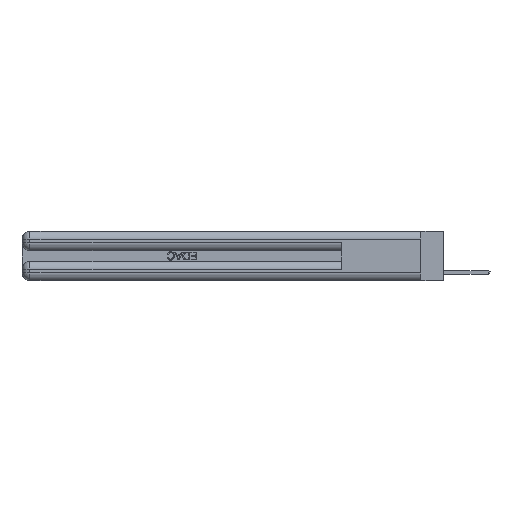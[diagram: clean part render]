
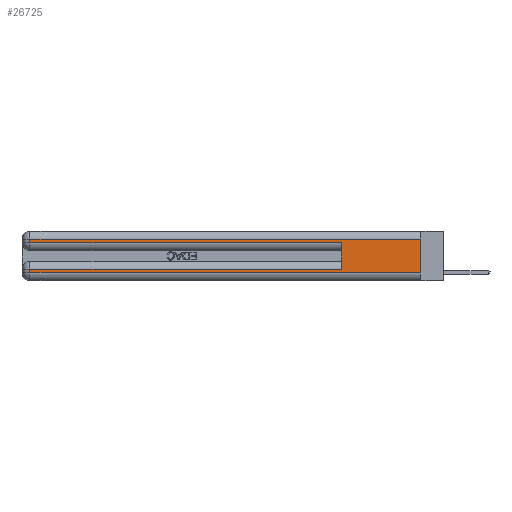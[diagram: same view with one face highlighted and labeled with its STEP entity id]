
A CAD part, left-side view. The second image highlights one B-rep face of the part: STEP entity #26725.
In plain terms, the highlighted planar face has unit normal (-1, 0, 0).
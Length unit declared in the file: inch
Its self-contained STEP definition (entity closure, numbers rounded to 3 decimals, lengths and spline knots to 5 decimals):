
#1378 = ORIENTED_EDGE ( 'NONE', *, *, #25001, .T. ) ;
#1379 = CARTESIAN_POINT ( 'NONE',  ( 0., 2.94, 0.06 ) ) ;
#1670 = ORIENTED_EDGE ( 'NONE', *, *, #17466, .T. ) ;
#1953 = VECTOR ( 'NONE', #6550, 39.37008 ) ;
#2352 = VERTEX_POINT ( 'NONE', #7837 ) ;
#2622 = DIRECTION ( 'NONE',  ( 0., 0., -1. ) ) ;
#2938 = PLANE ( 'NONE',  #23205 ) ;
#3796 = CARTESIAN_POINT ( 'NONE',  ( 0., 2.94, 0.31 ) ) ;
#4216 = VERTEX_POINT ( 'NONE', #20853 ) ;
#4381 = ORIENTED_EDGE ( 'NONE', *, *, #17596, .T. ) ;
#4648 = EDGE_CURVE ( 'NONE', #2352, #10303, #21858, .T. ) ;
#4790 = DIRECTION ( 'NONE',  ( 0., 0., -1. ) ) ;
#4871 = CARTESIAN_POINT ( 'NONE',  ( 0., 0., 0.37 ) ) ;
#5040 = ORIENTED_EDGE ( 'NONE', *, *, #4648, .T. ) ;
#5120 = LINE ( 'NONE', #5767, #29321 ) ;
#5767 = CARTESIAN_POINT ( 'NONE',  ( 0., 0., 0.06 ) ) ;
#6040 = VERTEX_POINT ( 'NONE', #1379 ) ;
#6550 = DIRECTION ( 'NONE',  ( 0., -1., 0. ) ) ;
#7837 = CARTESIAN_POINT ( 'NONE',  ( 0., 0., 0.31 ) ) ;
#8303 = VECTOR ( 'NONE', #22413, 39.37008 ) ;
#8618 = CARTESIAN_POINT ( 'NONE',  ( 0., 0., 0.085 ) ) ;
#8828 = CARTESIAN_POINT ( 'NONE',  ( 0., 2.94, 0.085 ) ) ;
#8985 = EDGE_LOOP ( 'NONE', ( #27594, #5040, #1378, #4381, #17745, #23721, #13325, #1670 ) ) ;
#10303 = VERTEX_POINT ( 'NONE', #3796 ) ;
#10445 = LINE ( 'NONE', #4871, #27863 ) ;
#10473 = VERTEX_POINT ( 'NONE', #25720 ) ;
#10972 = CARTESIAN_POINT ( 'NONE',  ( 0., 2.94, 0.37 ) ) ;
#11190 = CARTESIAN_POINT ( 'NONE',  ( 0., 0., 0.31 ) ) ;
#12727 = VECTOR ( 'NONE', #4790, 39.37008 ) ;
#13325 = ORIENTED_EDGE ( 'NONE', *, *, #14059, .T. ) ;
#14059 = EDGE_CURVE ( 'NONE', #20688, #6040, #20283, .T. ) ;
#15832 = CARTESIAN_POINT ( 'NONE',  ( 0., 0.6, 0.145 ) ) ;
#16361 = DIRECTION ( 'NONE',  ( 0., 0., -1. ) ) ;
#16920 = DIRECTION ( 'NONE',  ( 0., 0., -1. ) ) ;
#17236 = FACE_OUTER_BOUND ( 'NONE', #8985, .T. ) ;
#17356 = VERTEX_POINT ( 'NONE', #28339 ) ;
#17358 = LINE ( 'NONE', #10972, #12727 ) ;
#17466 = EDGE_CURVE ( 'NONE', #6040, #4216, #5120, .T. ) ;
#17596 = EDGE_CURVE ( 'NONE', #18156, #17356, #19018, .T. ) ;
#17745 = ORIENTED_EDGE ( 'NONE', *, *, #18530, .F. ) ;
#18156 = VERTEX_POINT ( 'NONE', #21654 ) ;
#18445 = EDGE_CURVE ( 'NONE', #10473, #20688, #26101, .T. ) ;
#18530 = EDGE_CURVE ( 'NONE', #10473, #17356, #23618, .T. ) ;
#19018 = LINE ( 'NONE', #25165, #1953 ) ;
#19565 = VECTOR ( 'NONE', #16920, 39.37008 ) ;
#19638 = CARTESIAN_POINT ( 'NONE',  ( 0., 2.94, 0.37 ) ) ;
#19716 = DIRECTION ( 'NONE',  ( 0., -1., 0. ) ) ;
#20283 = LINE ( 'NONE', #19638, #19565 ) ;
#20688 = VERTEX_POINT ( 'NONE', #8828 ) ;
#20853 = CARTESIAN_POINT ( 'NONE',  ( 0., 0., 0.06 ) ) ;
#21237 = EDGE_CURVE ( 'NONE', #2352, #4216, #10445, .T. ) ;
#21654 = CARTESIAN_POINT ( 'NONE',  ( 0., 2.94, 0.285 ) ) ;
#21858 = LINE ( 'NONE', #11190, #24322 ) ;
#22413 = DIRECTION ( 'NONE',  ( 0., 1., 0. ) ) ;
#23205 = AXIS2_PLACEMENT_3D ( 'NONE', #25722, #25823, #16361 ) ;
#23618 = LINE ( 'NONE', #15832, #27465 ) ;
#23721 = ORIENTED_EDGE ( 'NONE', *, *, #18445, .T. ) ;
#24322 = VECTOR ( 'NONE', #29281, 39.37008 ) ;
#24892 = DIRECTION ( 'NONE',  ( 0., 0., 1. ) ) ;
#25001 = EDGE_CURVE ( 'NONE', #10303, #18156, #17358, .T. ) ;
#25165 = CARTESIAN_POINT ( 'NONE',  ( 0., 0., 0.285 ) ) ;
#25720 = CARTESIAN_POINT ( 'NONE',  ( 0., 0.6, 0.085 ) ) ;
#25722 = CARTESIAN_POINT ( 'NONE',  ( 0., 0., 0.37 ) ) ;
#25823 = DIRECTION ( 'NONE',  ( 1., 0., 0. ) ) ;
#26101 = LINE ( 'NONE', #8618, #8303 ) ;
#26725 = ADVANCED_FACE ( 'NONE', ( #17236 ), #2938, .F. ) ;
#27465 = VECTOR ( 'NONE', #24892, 39.37008 ) ;
#27594 = ORIENTED_EDGE ( 'NONE', *, *, #21237, .F. ) ;
#27863 = VECTOR ( 'NONE', #2622, 39.37008 ) ;
#28339 = CARTESIAN_POINT ( 'NONE',  ( 0., 0.6, 0.285 ) ) ;
#29281 = DIRECTION ( 'NONE',  ( 0., 1., 0. ) ) ;
#29321 = VECTOR ( 'NONE', #19716, 39.37008 ) ;
